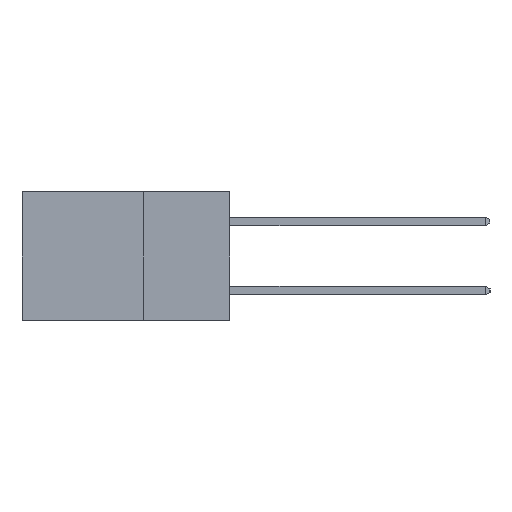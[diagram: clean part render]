
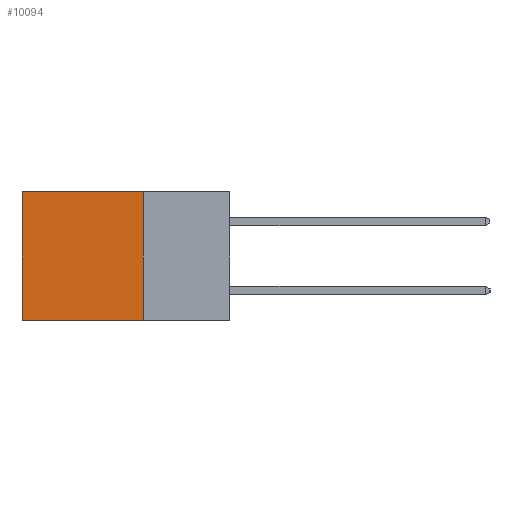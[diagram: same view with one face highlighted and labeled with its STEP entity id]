
A CAD part, left-side view. The second image highlights one B-rep face of the part: STEP entity #10094.
In plain terms, the highlighted planar face has unit normal (-1, 0, 0).
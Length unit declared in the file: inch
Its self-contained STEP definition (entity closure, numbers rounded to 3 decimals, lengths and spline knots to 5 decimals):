
#344 = CARTESIAN_POINT ( 'NONE',  ( 0.2615, 0.6, 0. ) ) ;
#377 = DIRECTION ( 'NONE',  ( 0., 0., -1. ) ) ;
#538 = VERTEX_POINT ( 'NONE', #584 ) ;
#584 = CARTESIAN_POINT ( 'NONE',  ( 0.2615, 0.6, -0.37 ) ) ;
#790 = DIRECTION ( 'NONE',  ( 0., 1., 0. ) ) ;
#835 = VECTOR ( 'NONE', #3801, 39.37008 ) ;
#957 = CARTESIAN_POINT ( 'NONE',  ( 0.2615, 0.25, 0. ) ) ;
#1134 = LINE ( 'NONE', #6782, #835 ) ;
#1174 = DIRECTION ( 'NONE',  ( 1., 0., 0. ) ) ;
#1382 = ORIENTED_EDGE ( 'NONE', *, *, #9470, .F. ) ;
#1437 = EDGE_CURVE ( 'NONE', #1911, #11381, #8170, .T. ) ;
#1823 = VERTEX_POINT ( 'NONE', #4055 ) ;
#1911 = VERTEX_POINT ( 'NONE', #8948 ) ;
#2048 = VECTOR ( 'NONE', #7519, 39.37008 ) ;
#2386 = EDGE_CURVE ( 'NONE', #1823, #538, #4384, .T. ) ;
#3076 = CARTESIAN_POINT ( 'NONE',  ( 0.2615, 0.25, -0.37 ) ) ;
#3207 = ORIENTED_EDGE ( 'NONE', *, *, #5008, .T. ) ;
#3376 = CARTESIAN_POINT ( 'NONE',  ( 0.2615, 0.25, -0.37 ) ) ;
#3551 = VECTOR ( 'NONE', #790, 39.37008 ) ;
#3801 = DIRECTION ( 'NONE',  ( 0., 0., -1. ) ) ;
#4055 = CARTESIAN_POINT ( 'NONE',  ( 0.2615, 0.25, -0.37 ) ) ;
#4357 = EDGE_LOOP ( 'NONE', ( #3207, #5503, #1382, #10711 ) ) ;
#4384 = LINE ( 'NONE', #3376, #2048 ) ;
#4523 = LINE ( 'NONE', #3076, #10962 ) ;
#4692 = CARTESIAN_POINT ( 'NONE',  ( 0.2615, 0.25, -0.37 ) ) ;
#5008 = EDGE_CURVE ( 'NONE', #11381, #538, #1134, .T. ) ;
#5503 = ORIENTED_EDGE ( 'NONE', *, *, #2386, .F. ) ;
#6429 = PLANE ( 'NONE',  #6602 ) ;
#6602 = AXIS2_PLACEMENT_3D ( 'NONE', #4692, #1174, #7302 ) ;
#6782 = CARTESIAN_POINT ( 'NONE',  ( 0.2615, 0.6, -0.37 ) ) ;
#6923 = FACE_OUTER_BOUND ( 'NONE', #4357, .T. ) ;
#7302 = DIRECTION ( 'NONE',  ( 0., 0., -1. ) ) ;
#7519 = DIRECTION ( 'NONE',  ( 0., 1., 0. ) ) ;
#8170 = LINE ( 'NONE', #957, #3551 ) ;
#8948 = CARTESIAN_POINT ( 'NONE',  ( 0.2615, 0.25, 0. ) ) ;
#9470 = EDGE_CURVE ( 'NONE', #1911, #1823, #4523, .T. ) ;
#10094 = ADVANCED_FACE ( 'NONE', ( #6923 ), #6429, .F. ) ;
#10711 = ORIENTED_EDGE ( 'NONE', *, *, #1437, .T. ) ;
#10962 = VECTOR ( 'NONE', #377, 39.37008 ) ;
#11381 = VERTEX_POINT ( 'NONE', #344 ) ;
